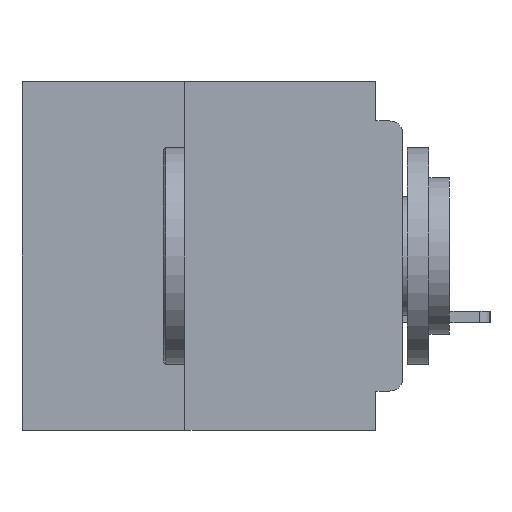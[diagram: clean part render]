
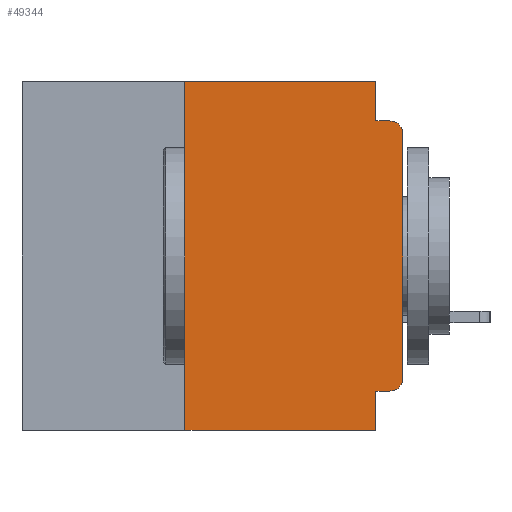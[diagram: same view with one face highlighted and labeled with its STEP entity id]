
A CAD part, left-side view. The second image highlights one B-rep face of the part: STEP entity #49344.
In plain terms, the highlighted planar face has unit normal (-1, 0, 0).
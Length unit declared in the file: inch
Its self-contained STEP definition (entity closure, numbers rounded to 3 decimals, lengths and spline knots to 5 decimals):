
#934 = CARTESIAN_POINT ( 'NONE',  ( 0., 0.031, 0. ) ) ;
#1448 = CARTESIAN_POINT ( 'NONE',  ( 0., 0., -0.045 ) ) ;
#1632 = FACE_OUTER_BOUND ( 'NONE', #8052, .T. ) ;
#2268 = EDGE_CURVE ( 'NONE', #30202, #38274, #24367, .T. ) ;
#3306 = VERTEX_POINT ( 'NONE', #43843 ) ;
#3739 = CARTESIAN_POINT ( 'NONE',  ( 0., 0., -0.34 ) ) ;
#4579 = VECTOR ( 'NONE', #22379, 39.37008 ) ;
#5044 = DIRECTION ( 'NONE',  ( 0., 0., -1. ) ) ;
#5566 = VERTEX_POINT ( 'NONE', #37394 ) ;
#7668 = VERTEX_POINT ( 'NONE', #38634 ) ;
#8052 = EDGE_LOOP ( 'NONE', ( #30647, #29686, #18201, #21786, #23656, #15915, #45818, #17062, #26535, #47544 ) ) ;
#8292 = DIRECTION ( 'NONE',  ( -1., 0., 0. ) ) ;
#8358 = EDGE_CURVE ( 'NONE', #38060, #27479, #26899, .T. ) ;
#9150 = LINE ( 'NONE', #1448, #20281 ) ;
#9314 = CARTESIAN_POINT ( 'NONE',  ( 0., 0.437, -0.4 ) ) ;
#9778 = DIRECTION ( 'NONE',  ( 0., -1., 0. ) ) ;
#9796 = CARTESIAN_POINT ( 'NONE',  ( 0., 0.437, 0. ) ) ;
#12897 = EDGE_CURVE ( 'NONE', #51165, #5566, #9150, .T. ) ;
#13213 = DIRECTION ( 'NONE',  ( 0., 0., 1. ) ) ;
#15032 = LINE ( 'NONE', #50674, #35695 ) ;
#15582 = CARTESIAN_POINT ( 'NONE',  ( 0., 0.25, -0.4 ) ) ;
#15656 = AXIS2_PLACEMENT_3D ( 'NONE', #43180, #18610, #47317 ) ;
#15915 = ORIENTED_EDGE ( 'NONE', *, *, #19150, .F. ) ;
#17062 = ORIENTED_EDGE ( 'NONE', *, *, #50424, .F. ) ;
#18201 = ORIENTED_EDGE ( 'NONE', *, *, #12897, .F. ) ;
#18610 = DIRECTION ( 'NONE',  ( -1., 0., 0. ) ) ;
#19150 = EDGE_CURVE ( 'NONE', #30202, #3306, #21187, .T. ) ;
#20281 = VECTOR ( 'NONE', #34723, 39.37008 ) ;
#21187 = LINE ( 'NONE', #50305, #32122 ) ;
#21262 = LINE ( 'NONE', #31750, #41769 ) ;
#21786 = ORIENTED_EDGE ( 'NONE', *, *, #21935, .F. ) ;
#21935 = EDGE_CURVE ( 'NONE', #7668, #51165, #52357, .T. ) ;
#22014 = EDGE_CURVE ( 'NONE', #3306, #7668, #48526, .T. ) ;
#22379 = DIRECTION ( 'NONE',  ( 0., -1., 0. ) ) ;
#22503 = VERTEX_POINT ( 'NONE', #50263 ) ;
#23073 = VECTOR ( 'NONE', #9778, 39.37008 ) ;
#23593 = DIRECTION ( 'NONE',  ( 0., 0., -1. ) ) ;
#23656 = ORIENTED_EDGE ( 'NONE', *, *, #22014, .F. ) ;
#24367 = LINE ( 'NONE', #9314, #23073 ) ;
#25069 = EDGE_CURVE ( 'NONE', #22503, #5566, #51891, .T. ) ;
#25301 = LINE ( 'NONE', #53378, #47105 ) ;
#26535 = ORIENTED_EDGE ( 'NONE', *, *, #44296, .F. ) ;
#26899 = CIRCLE ( 'NONE', #52494, 0.015 ) ;
#27479 = VERTEX_POINT ( 'NONE', #3739 ) ;
#27886 = VERTEX_POINT ( 'NONE', #51903 ) ;
#28810 = DIRECTION ( 'NONE',  ( 0., 0., 1. ) ) ;
#29686 = ORIENTED_EDGE ( 'NONE', *, *, #25069, .T. ) ;
#30202 = VERTEX_POINT ( 'NONE', #15582 ) ;
#30593 = VECTOR ( 'NONE', #5044, 39.37008 ) ;
#30647 = ORIENTED_EDGE ( 'NONE', *, *, #46028, .T. ) ;
#31750 = CARTESIAN_POINT ( 'NONE',  ( 0., 0.031, -0.4 ) ) ;
#32122 = VECTOR ( 'NONE', #13213, 39.37008 ) ;
#33111 = CARTESIAN_POINT ( 'NONE',  ( 0., 0.015, -0.34 ) ) ;
#34723 = DIRECTION ( 'NONE',  ( 0., -1., 0. ) ) ;
#35695 = VECTOR ( 'NONE', #42608, 39.37008 ) ;
#35821 = AXIS2_PLACEMENT_3D ( 'NONE', #47965, #48132, #23593 ) ;
#35857 = DIRECTION ( 'NONE',  ( 0., 0., -1. ) ) ;
#37210 = DIRECTION ( 'NONE',  ( 0., 0., -1. ) ) ;
#37394 = CARTESIAN_POINT ( 'NONE',  ( 0., 0.015, -0.045 ) ) ;
#38060 = VERTEX_POINT ( 'NONE', #45130 ) ;
#38128 = CARTESIAN_POINT ( 'NONE',  ( 0., 0.031, -0.4 ) ) ;
#38274 = VERTEX_POINT ( 'NONE', #38128 ) ;
#38634 = CARTESIAN_POINT ( 'NONE',  ( 0., 0.031, 0. ) ) ;
#41769 = VECTOR ( 'NONE', #35857, 39.37008 ) ;
#42608 = DIRECTION ( 'NONE',  ( 0., 1., 0. ) ) ;
#42867 = CARTESIAN_POINT ( 'NONE',  ( 0., 0.031, -0.045 ) ) ;
#43180 = CARTESIAN_POINT ( 'NONE',  ( 0., 0.015, -0.06 ) ) ;
#43843 = CARTESIAN_POINT ( 'NONE',  ( 0., 0.25, 0. ) ) ;
#44016 = PLANE ( 'NONE',  #35821 ) ;
#44296 = EDGE_CURVE ( 'NONE', #38060, #27886, #15032, .T. ) ;
#45130 = CARTESIAN_POINT ( 'NONE',  ( 0., 0.015, -0.355 ) ) ;
#45818 = ORIENTED_EDGE ( 'NONE', *, *, #2268, .T. ) ;
#46028 = EDGE_CURVE ( 'NONE', #27479, #22503, #25301, .T. ) ;
#47105 = VECTOR ( 'NONE', #28810, 39.37008 ) ;
#47317 = DIRECTION ( 'NONE',  ( 0., 0., -1. ) ) ;
#47544 = ORIENTED_EDGE ( 'NONE', *, *, #8358, .T. ) ;
#47965 = CARTESIAN_POINT ( 'NONE',  ( 0., 0.437, 0. ) ) ;
#48132 = DIRECTION ( 'NONE',  ( 1., 0., 0. ) ) ;
#48526 = LINE ( 'NONE', #9796, #4579 ) ;
#49344 = ADVANCED_FACE ( 'NONE', ( #1632 ), #44016, .F. ) ;
#50263 = CARTESIAN_POINT ( 'NONE',  ( 0., 0., -0.06 ) ) ;
#50305 = CARTESIAN_POINT ( 'NONE',  ( 0., 0.25, -0.4 ) ) ;
#50424 = EDGE_CURVE ( 'NONE', #27886, #38274, #21262, .T. ) ;
#50674 = CARTESIAN_POINT ( 'NONE',  ( 0., 0., -0.355 ) ) ;
#51165 = VERTEX_POINT ( 'NONE', #42867 ) ;
#51891 = CIRCLE ( 'NONE', #15656, 0.015 ) ;
#51903 = CARTESIAN_POINT ( 'NONE',  ( 0., 0.031, -0.355 ) ) ;
#52357 = LINE ( 'NONE', #934, #30593 ) ;
#52494 = AXIS2_PLACEMENT_3D ( 'NONE', #33111, #8292, #37210 ) ;
#53378 = CARTESIAN_POINT ( 'NONE',  ( 0., 0., 0. ) ) ;
